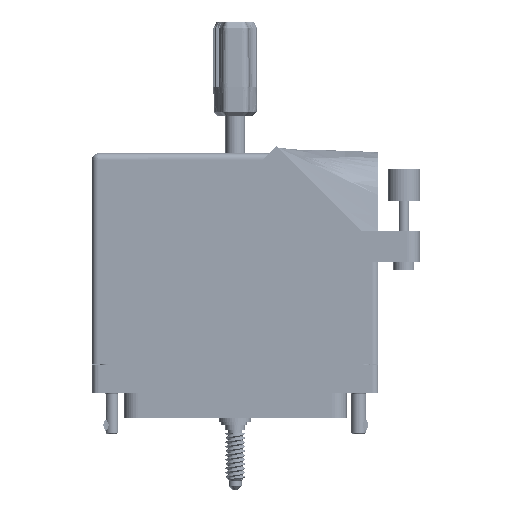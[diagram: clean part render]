
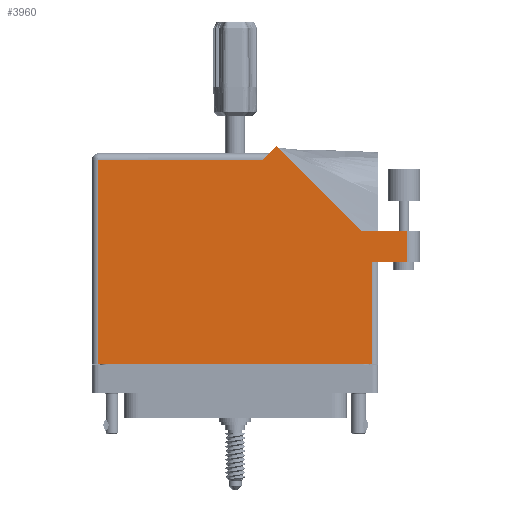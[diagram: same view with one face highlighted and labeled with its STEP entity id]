
A CAD part, front view. The second image highlights one B-rep face of the part: STEP entity #3960.
In plain terms, the highlighted face is planar.
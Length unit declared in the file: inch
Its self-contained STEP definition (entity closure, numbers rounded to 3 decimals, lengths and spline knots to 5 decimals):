
#2644 = DIRECTION ( 'NONE',  ( -1., 0., 0. ) ) ;
#3196 = LINE ( 'NONE', #56261, #115243 ) ;
#3960 = ADVANCED_FACE ( 'NONE', ( #82773 ), #22768, .F. ) ;
#4046 = ORIENTED_EDGE ( 'NONE', *, *, #37002, .T. ) ;
#4323 = ORIENTED_EDGE ( 'NONE', *, *, #61383, .T. ) ;
#5477 = CARTESIAN_POINT ( 'NONE',  ( 1.3155, -0.1, 0.765 ) ) ;
#8791 = LINE ( 'NONE', #100077, #29610 ) ;
#9162 = VERTEX_POINT ( 'NONE', #5477 ) ;
#13211 = CARTESIAN_POINT ( 'NONE',  ( -1.3775, -0.1, 0.765 ) ) ;
#14589 = CARTESIAN_POINT ( 'NONE',  ( -1.3775, 1.93, 0.765 ) ) ;
#15313 = CARTESIAN_POINT ( 'NONE',  ( -1.3155, -0.1, 0.765 ) ) ;
#15411 = DIRECTION ( 'NONE',  ( 0., 1., 0. ) ) ;
#16374 = ORIENTED_EDGE ( 'NONE', *, *, #76081, .T. ) ;
#19073 = LINE ( 'NONE', #88223, #115747 ) ;
#22768 = PLANE ( 'NONE',  #109491 ) ;
#23548 = DIRECTION ( 'NONE',  ( -1., 0., 0. ) ) ;
#25726 = VECTOR ( 'NONE', #73161, 39.37008 ) ;
#26139 = ORIENTED_EDGE ( 'NONE', *, *, #103428, .T. ) ;
#26347 = ORIENTED_EDGE ( 'NONE', *, *, #48471, .T. ) ;
#27752 = VERTEX_POINT ( 'NONE', #15313 ) ;
#28473 = DIRECTION ( 'NONE',  ( 1., 0., 0. ) ) ;
#29610 = VECTOR ( 'NONE', #28473, 39.37008 ) ;
#30490 = CARTESIAN_POINT ( 'NONE',  ( 0.2655, 1.868, 0.765 ) ) ;
#31953 = LINE ( 'NONE', #98866, #111782 ) ;
#33353 = VECTOR ( 'NONE', #39401, 39.37008 ) ;
#33877 = VERTEX_POINT ( 'NONE', #84734 ) ;
#35884 = CARTESIAN_POINT ( 'NONE',  ( -1.3155, 1.868, 0.765 ) ) ;
#37002 = EDGE_CURVE ( 'NONE', #33877, #91666, #8791, .T. ) ;
#37529 = EDGE_CURVE ( 'NONE', #27752, #9162, #51591, .T. ) ;
#38097 = LINE ( 'NONE', #63197, #39427 ) ;
#39401 = DIRECTION ( 'NONE',  ( 1., 0., 0. ) ) ;
#39427 = VECTOR ( 'NONE', #15411, 39.37008 ) ;
#39941 = LINE ( 'NONE', #46262, #62521 ) ;
#41856 = EDGE_CURVE ( 'NONE', #44303, #100677, #3196, .T. ) ;
#43142 = ORIENTED_EDGE ( 'NONE', *, *, #37529, .T. ) ;
#43169 = ORIENTED_EDGE ( 'NONE', *, *, #79963, .T. ) ;
#43743 = DIRECTION ( 'NONE',  ( 0., 1., 0. ) ) ;
#44303 = VERTEX_POINT ( 'NONE', #30490 ) ;
#44754 = VERTEX_POINT ( 'NONE', #78182 ) ;
#46146 = VERTEX_POINT ( 'NONE', #84588 ) ;
#46262 = CARTESIAN_POINT ( 'NONE',  ( 1.7775, 1.187, 0.765 ) ) ;
#48471 = EDGE_CURVE ( 'NONE', #44754, #44303, #31953, .T. ) ;
#51591 = LINE ( 'NONE', #13211, #33353 ) ;
#55309 = ORIENTED_EDGE ( 'NONE', *, *, #41856, .T. ) ;
#55380 = DIRECTION ( 'NONE',  ( -1., 0., 0. ) ) ;
#56261 = CARTESIAN_POINT ( 'NONE',  ( -1.3775, 1.868, 0.765 ) ) ;
#60860 = LINE ( 'NONE', #109856, #25726 ) ;
#61383 = EDGE_CURVE ( 'NONE', #100677, #27752, #60860, .T. ) ;
#62521 = VECTOR ( 'NONE', #55380, 39.37008 ) ;
#63197 = CARTESIAN_POINT ( 'NONE',  ( 1.6525, 1.187, 0.765 ) ) ;
#66303 = LINE ( 'NONE', #79853, #105397 ) ;
#73161 = DIRECTION ( 'NONE',  ( 0., -1., 0. ) ) ;
#76081 = EDGE_CURVE ( 'NONE', #108384, #44754, #19073, .T. ) ;
#77271 = DIRECTION ( 'NONE',  ( 0., 0., -1. ) ) ;
#78182 = CARTESIAN_POINT ( 'NONE',  ( 0.39821, 2.00071, 0.765 ) ) ;
#79853 = CARTESIAN_POINT ( 'NONE',  ( 1.3155, 0.88, 0.765 ) ) ;
#79963 = EDGE_CURVE ( 'NONE', #91666, #46146, #38097, .T. ) ;
#82773 = FACE_OUTER_BOUND ( 'NONE', #113234, .T. ) ;
#84588 = CARTESIAN_POINT ( 'NONE',  ( 1.6525, 1.187, 0.765 ) ) ;
#84734 = CARTESIAN_POINT ( 'NONE',  ( 1.3155, 0.88, 0.765 ) ) ;
#88223 = CARTESIAN_POINT ( 'NONE',  ( 1.21192, 1.187, 0.765 ) ) ;
#91666 = VERTEX_POINT ( 'NONE', #93297 ) ;
#93297 = CARTESIAN_POINT ( 'NONE',  ( 1.6525, 0.88, 0.765 ) ) ;
#97363 = DIRECTION ( 'NONE',  ( -0.707, -0.707, 0. ) ) ;
#97592 = DIRECTION ( 'NONE',  ( -0.707, 0.707, 0. ) ) ;
#98866 = CARTESIAN_POINT ( 'NONE',  ( 0.3275, 1.93, 0.765 ) ) ;
#100077 = CARTESIAN_POINT ( 'NONE',  ( 1.3775, 0.88, 0.765 ) ) ;
#100677 = VERTEX_POINT ( 'NONE', #35884 ) ;
#103428 = EDGE_CURVE ( 'NONE', #9162, #33877, #66303, .T. ) ;
#105397 = VECTOR ( 'NONE', #43743, 39.37008 ) ;
#106003 = EDGE_CURVE ( 'NONE', #46146, #108384, #39941, .T. ) ;
#108384 = VERTEX_POINT ( 'NONE', #114567 ) ;
#109491 = AXIS2_PLACEMENT_3D ( 'NONE', #14589, #77271, #23548 ) ;
#109856 = CARTESIAN_POINT ( 'NONE',  ( -1.3155, -0.1, 0.765 ) ) ;
#110159 = ORIENTED_EDGE ( 'NONE', *, *, #106003, .T. ) ;
#111782 = VECTOR ( 'NONE', #97363, 39.37008 ) ;
#113234 = EDGE_LOOP ( 'NONE', ( #4046, #43169, #110159, #16374, #26347, #55309, #4323, #43142, #26139 ) ) ;
#114567 = CARTESIAN_POINT ( 'NONE',  ( 1.21192, 1.187, 0.765 ) ) ;
#115243 = VECTOR ( 'NONE', #2644, 39.37008 ) ;
#115747 = VECTOR ( 'NONE', #97592, 39.37008 ) ;
